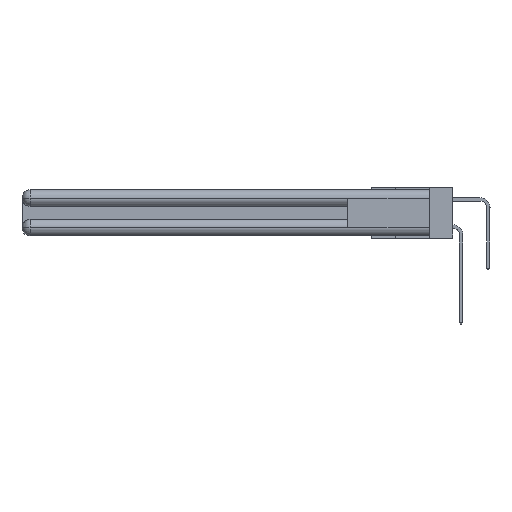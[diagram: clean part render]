
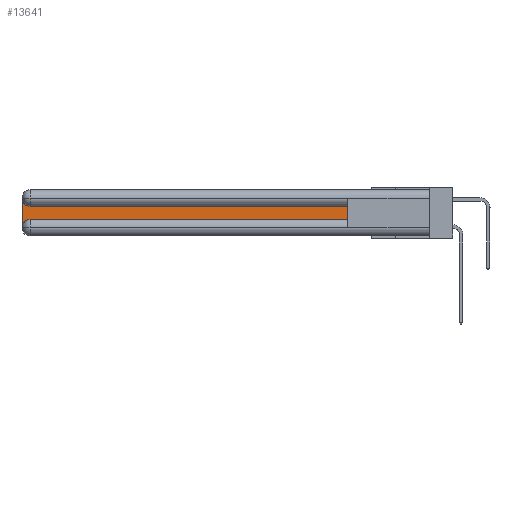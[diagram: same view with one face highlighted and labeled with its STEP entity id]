
A CAD part, left-side view. The second image highlights one B-rep face of the part: STEP entity #13641.
In plain terms, the highlighted planar face has unit normal (-1, 0, 0).
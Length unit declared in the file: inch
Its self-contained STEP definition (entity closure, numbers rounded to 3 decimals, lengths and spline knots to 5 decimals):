
#215 = CARTESIAN_POINT ( 'NONE',  ( 0.075, 3., -0.2175 ) ) ;
#734 = EDGE_CURVE ( 'NONE', #21322, #1724, #1960, .T. ) ;
#1084 = DIRECTION ( 'NONE',  ( 0., 0., -1. ) ) ;
#1724 = VERTEX_POINT ( 'NONE', #13388 ) ;
#1960 = LINE ( 'NONE', #12872, #30008 ) ;
#3060 = DIRECTION ( 'NONE',  ( 0., 0., -1. ) ) ;
#4155 = ORIENTED_EDGE ( 'NONE', *, *, #734, .T. ) ;
#4689 = AXIS2_PLACEMENT_3D ( 'NONE', #19986, #22716, #33069 ) ;
#5148 = DIRECTION ( 'NONE',  ( 0., 1., 0. ) ) ;
#6319 = CARTESIAN_POINT ( 'NONE',  ( 0.075, 2.94, -0.0625 ) ) ;
#6786 = ORIENTED_EDGE ( 'NONE', *, *, #25751, .T. ) ;
#6971 = PLANE ( 'NONE',  #15622 ) ;
#7700 = DIRECTION ( 'NONE',  ( 0., -1., 0. ) ) ;
#9036 = CARTESIAN_POINT ( 'NONE',  ( 0.075, 0.6, -0.2175 ) ) ;
#9433 = CARTESIAN_POINT ( 'NONE',  ( 0.075, 3., -0.2775 ) ) ;
#9717 = DIRECTION ( 'NONE',  ( 0., 0., -1. ) ) ;
#10950 = EDGE_CURVE ( 'NONE', #32349, #21322, #22689, .T. ) ;
#12260 = DIRECTION ( 'NONE',  ( 1., 0., 0. ) ) ;
#12569 = EDGE_CURVE ( 'NONE', #34247, #32349, #32843, .T. ) ;
#12759 = CIRCLE ( 'NONE', #18068, 0.06 ) ;
#12872 = CARTESIAN_POINT ( 'NONE',  ( 0.075, 0.6, -0.1225 ) ) ;
#13388 = CARTESIAN_POINT ( 'NONE',  ( 0.075, 2.94, -0.1225 ) ) ;
#13641 = ADVANCED_FACE ( 'NONE', ( #28154 ), #6971, .F. ) ;
#14036 = EDGE_CURVE ( 'NONE', #33891, #32683, #16686, .T. ) ;
#15622 = AXIS2_PLACEMENT_3D ( 'NONE', #18150, #23273, #9717 ) ;
#16172 = CARTESIAN_POINT ( 'NONE',  ( 0.075, 0.6, -0.1225 ) ) ;
#16601 = CARTESIAN_POINT ( 'NONE',  ( 0.075, 3., -0.0625 ) ) ;
#16686 = LINE ( 'NONE', #215, #27719 ) ;
#18068 = AXIS2_PLACEMENT_3D ( 'NONE', #6319, #12260, #1084 ) ;
#18150 = CARTESIAN_POINT ( 'NONE',  ( 0.075, 3., -0.1225 ) ) ;
#18206 = ORIENTED_EDGE ( 'NONE', *, *, #34799, .T. ) ;
#19986 = CARTESIAN_POINT ( 'NONE',  ( 0.075, 2.94, -0.2775 ) ) ;
#20849 = EDGE_LOOP ( 'NONE', ( #4155, #18206, #26529, #6786, #27611, #23826 ) ) ;
#21322 = VERTEX_POINT ( 'NONE', #16172 ) ;
#22689 = LINE ( 'NONE', #9036, #26962 ) ;
#22716 = DIRECTION ( 'NONE',  ( 1., 0., 0. ) ) ;
#23273 = DIRECTION ( 'NONE',  ( 1., 0., 0. ) ) ;
#23598 = CARTESIAN_POINT ( 'NONE',  ( 0.075, 0.6, -0.2175 ) ) ;
#23826 = ORIENTED_EDGE ( 'NONE', *, *, #10950, .T. ) ;
#25053 = CIRCLE ( 'NONE', #4689, 0.06 ) ;
#25751 = EDGE_CURVE ( 'NONE', #32683, #34247, #25053, .T. ) ;
#26488 = CARTESIAN_POINT ( 'NONE',  ( 0.075, 0.6, -0.2175 ) ) ;
#26529 = ORIENTED_EDGE ( 'NONE', *, *, #14036, .T. ) ;
#26962 = VECTOR ( 'NONE', #33903, 39.37008 ) ;
#27611 = ORIENTED_EDGE ( 'NONE', *, *, #12569, .T. ) ;
#27719 = VECTOR ( 'NONE', #3060, 39.37008 ) ;
#28154 = FACE_OUTER_BOUND ( 'NONE', #20849, .T. ) ;
#28805 = CARTESIAN_POINT ( 'NONE',  ( 0.075, 2.94, -0.2175 ) ) ;
#28999 = VECTOR ( 'NONE', #7700, 39.37008 ) ;
#30008 = VECTOR ( 'NONE', #5148, 39.37008 ) ;
#32349 = VERTEX_POINT ( 'NONE', #23598 ) ;
#32683 = VERTEX_POINT ( 'NONE', #9433 ) ;
#32843 = LINE ( 'NONE', #26488, #28999 ) ;
#33069 = DIRECTION ( 'NONE',  ( 0., 0., -1. ) ) ;
#33891 = VERTEX_POINT ( 'NONE', #16601 ) ;
#33903 = DIRECTION ( 'NONE',  ( 0., 0., 1. ) ) ;
#34247 = VERTEX_POINT ( 'NONE', #28805 ) ;
#34799 = EDGE_CURVE ( 'NONE', #1724, #33891, #12759, .T. ) ;
